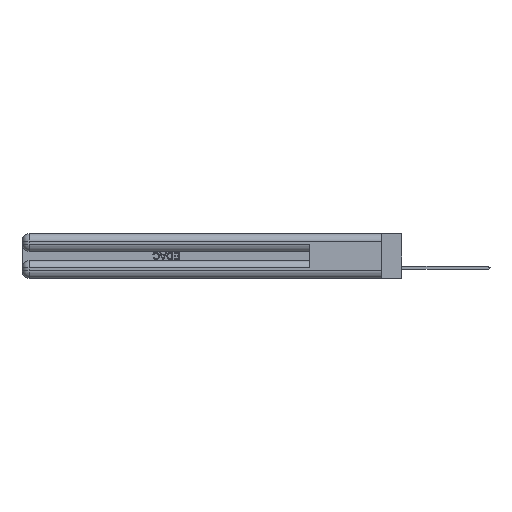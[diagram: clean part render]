
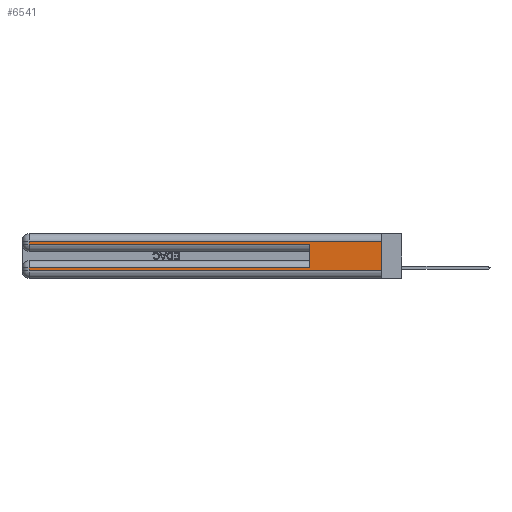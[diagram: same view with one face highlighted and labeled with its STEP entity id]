
A CAD part, left-side view. The second image highlights one B-rep face of the part: STEP entity #6541.
In plain terms, the highlighted planar face has unit normal (-1, 0, 0).
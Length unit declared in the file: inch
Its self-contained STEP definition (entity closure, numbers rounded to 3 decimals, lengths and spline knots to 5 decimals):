
#293 = VERTEX_POINT ( 'NONE', #31811 ) ;
#412 = CARTESIAN_POINT ( 'NONE',  ( 0., 2.94, 0.37 ) ) ;
#712 = DIRECTION ( 'NONE',  ( 0., 0., -1. ) ) ;
#1201 = CARTESIAN_POINT ( 'NONE',  ( 0., 0., 0.06 ) ) ;
#1455 = CARTESIAN_POINT ( 'NONE',  ( 0., 0., 0.285 ) ) ;
#2382 = CARTESIAN_POINT ( 'NONE',  ( 0., 0., 0.31 ) ) ;
#2785 = VECTOR ( 'NONE', #10445, 39.37008 ) ;
#3377 = LINE ( 'NONE', #34994, #36833 ) ;
#3569 = VECTOR ( 'NONE', #4958, 39.37008 ) ;
#3940 = VERTEX_POINT ( 'NONE', #2382 ) ;
#4209 = ORIENTED_EDGE ( 'NONE', *, *, #9901, .T. ) ;
#4886 = CARTESIAN_POINT ( 'NONE',  ( 0., 0., 0.37 ) ) ;
#4958 = DIRECTION ( 'NONE',  ( 0., -1., 0. ) ) ;
#5075 = EDGE_CURVE ( 'NONE', #3940, #31250, #3377, .T. ) ;
#6019 = ORIENTED_EDGE ( 'NONE', *, *, #27424, .T. ) ;
#6324 = VECTOR ( 'NONE', #38647, 39.37008 ) ;
#6541 = ADVANCED_FACE ( 'NONE', ( #9846 ), #17335, .F. ) ;
#6616 = CARTESIAN_POINT ( 'NONE',  ( 0., 0., 0.085 ) ) ;
#6774 = VERTEX_POINT ( 'NONE', #21356 ) ;
#6877 = ORIENTED_EDGE ( 'NONE', *, *, #14876, .T. ) ;
#8137 = CARTESIAN_POINT ( 'NONE',  ( 0., 2.94, 0.06 ) ) ;
#8144 = CARTESIAN_POINT ( 'NONE',  ( 0., 2.94, 0.285 ) ) ;
#8245 = CARTESIAN_POINT ( 'NONE',  ( 0., 0., 0.06 ) ) ;
#9190 = VERTEX_POINT ( 'NONE', #22203 ) ;
#9846 = FACE_OUTER_BOUND ( 'NONE', #32448, .T. ) ;
#9901 = EDGE_CURVE ( 'NONE', #293, #18429, #26499, .T. ) ;
#10445 = DIRECTION ( 'NONE',  ( 0., 1., 0. ) ) ;
#10857 = VECTOR ( 'NONE', #30497, 39.37008 ) ;
#10883 = CARTESIAN_POINT ( 'NONE',  ( 0., 0., 0.31 ) ) ;
#11837 = EDGE_CURVE ( 'NONE', #6774, #15978, #13350, .T. ) ;
#12060 = ORIENTED_EDGE ( 'NONE', *, *, #11837, .T. ) ;
#12533 = EDGE_CURVE ( 'NONE', #6774, #9190, #31211, .T. ) ;
#12666 = ORIENTED_EDGE ( 'NONE', *, *, #31013, .T. ) ;
#13350 = LINE ( 'NONE', #6616, #6324 ) ;
#14282 = LINE ( 'NONE', #10883, #2785 ) ;
#14876 = EDGE_CURVE ( 'NONE', #18429, #9190, #37538, .T. ) ;
#15978 = VERTEX_POINT ( 'NONE', #30036 ) ;
#15990 = DIRECTION ( 'NONE',  ( 0., 0., -1. ) ) ;
#16486 = LINE ( 'NONE', #8245, #10857 ) ;
#16670 = CARTESIAN_POINT ( 'NONE',  ( 0., 2.94, 0.37 ) ) ;
#16914 = DIRECTION ( 'NONE',  ( 0., 0., -1. ) ) ;
#16923 = ORIENTED_EDGE ( 'NONE', *, *, #5075, .F. ) ;
#17335 = PLANE ( 'NONE',  #25655 ) ;
#18429 = VERTEX_POINT ( 'NONE', #8144 ) ;
#19434 = CARTESIAN_POINT ( 'NONE',  ( 0., 0.6, 0.145 ) ) ;
#19701 = VERTEX_POINT ( 'NONE', #8137 ) ;
#20031 = VECTOR ( 'NONE', #16914, 39.37008 ) ;
#21022 = EDGE_CURVE ( 'NONE', #15978, #19701, #39023, .T. ) ;
#21356 = CARTESIAN_POINT ( 'NONE',  ( 0., 0.6, 0.085 ) ) ;
#22203 = CARTESIAN_POINT ( 'NONE',  ( 0., 0.6, 0.285 ) ) ;
#22717 = VECTOR ( 'NONE', #35379, 39.37008 ) ;
#23200 = ORIENTED_EDGE ( 'NONE', *, *, #21022, .T. ) ;
#23910 = VECTOR ( 'NONE', #712, 39.37008 ) ;
#25655 = AXIS2_PLACEMENT_3D ( 'NONE', #4886, #30065, #36346 ) ;
#26499 = LINE ( 'NONE', #16670, #23910 ) ;
#27424 = EDGE_CURVE ( 'NONE', #19701, #31250, #16486, .T. ) ;
#30036 = CARTESIAN_POINT ( 'NONE',  ( 0., 2.94, 0.085 ) ) ;
#30065 = DIRECTION ( 'NONE',  ( 1., 0., 0. ) ) ;
#30497 = DIRECTION ( 'NONE',  ( 0., -1., 0. ) ) ;
#31013 = EDGE_CURVE ( 'NONE', #3940, #293, #14282, .T. ) ;
#31211 = LINE ( 'NONE', #19434, #22717 ) ;
#31250 = VERTEX_POINT ( 'NONE', #1201 ) ;
#31811 = CARTESIAN_POINT ( 'NONE',  ( 0., 2.94, 0.31 ) ) ;
#32448 = EDGE_LOOP ( 'NONE', ( #16923, #12666, #4209, #6877, #39144, #12060, #23200, #6019 ) ) ;
#34994 = CARTESIAN_POINT ( 'NONE',  ( 0., 0., 0.37 ) ) ;
#35379 = DIRECTION ( 'NONE',  ( 0., 0., 1. ) ) ;
#36346 = DIRECTION ( 'NONE',  ( 0., 0., -1. ) ) ;
#36833 = VECTOR ( 'NONE', #15990, 39.37008 ) ;
#37538 = LINE ( 'NONE', #1455, #3569 ) ;
#38647 = DIRECTION ( 'NONE',  ( 0., 1., 0. ) ) ;
#39023 = LINE ( 'NONE', #412, #20031 ) ;
#39144 = ORIENTED_EDGE ( 'NONE', *, *, #12533, .F. ) ;
